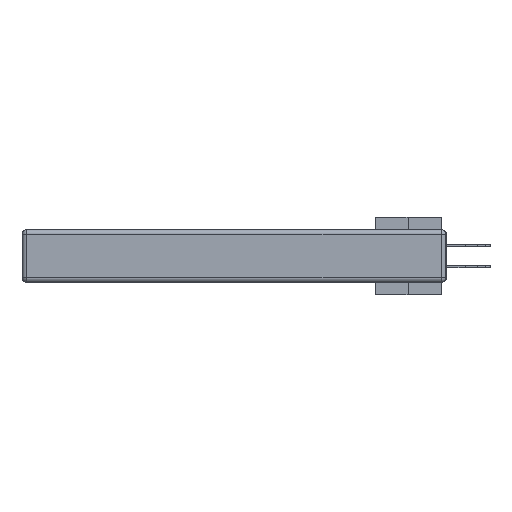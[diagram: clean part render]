
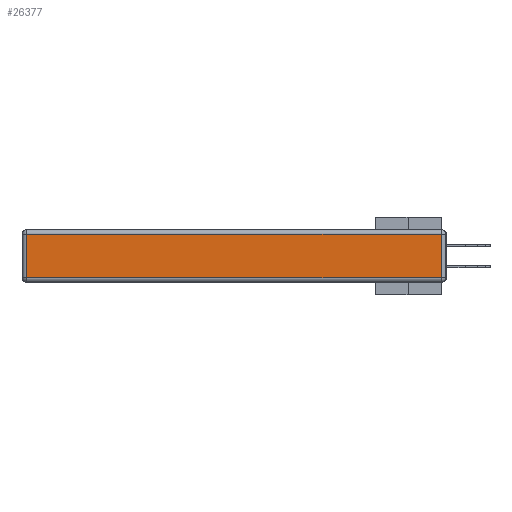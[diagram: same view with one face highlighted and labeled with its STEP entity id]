
A CAD part, left-side view. The second image highlights one B-rep face of the part: STEP entity #26377.
In plain terms, the highlighted planar face has unit normal (-1, 0, 0).
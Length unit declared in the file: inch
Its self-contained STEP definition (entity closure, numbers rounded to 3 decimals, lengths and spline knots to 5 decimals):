
#794 = EDGE_CURVE ( 'NONE', #29100, #9804, #16203, .T. ) ;
#1527 = CARTESIAN_POINT ( 'NONE',  ( 0., 2.75, -0.03 ) ) ;
#2427 = EDGE_LOOP ( 'NONE', ( #33691, #31388, #11139, #40716 ) ) ;
#3184 = CARTESIAN_POINT ( 'NONE',  ( 0., 2.72, -0.03 ) ) ;
#4443 = FACE_OUTER_BOUND ( 'NONE', #2427, .T. ) ;
#7871 = VERTEX_POINT ( 'NONE', #13119 ) ;
#8335 = LINE ( 'NONE', #18877, #35771 ) ;
#8372 = CARTESIAN_POINT ( 'NONE',  ( 0., 2.72, -0.313 ) ) ;
#9804 = VERTEX_POINT ( 'NONE', #3184 ) ;
#10887 = CARTESIAN_POINT ( 'NONE',  ( 0., 0.03, -0.03 ) ) ;
#11139 = ORIENTED_EDGE ( 'NONE', *, *, #794, .T. ) ;
#11229 = EDGE_CURVE ( 'NONE', #7871, #29100, #8335, .T. ) ;
#12417 = VECTOR ( 'NONE', #27567, 39.37008 ) ;
#13119 = CARTESIAN_POINT ( 'NONE',  ( 0., 0.03, -0.313 ) ) ;
#14620 = EDGE_CURVE ( 'NONE', #21224, #7871, #17449, .T. ) ;
#15185 = LINE ( 'NONE', #41942, #37026 ) ;
#16203 = LINE ( 'NONE', #1527, #41329 ) ;
#17449 = LINE ( 'NONE', #35045, #12417 ) ;
#18333 = CARTESIAN_POINT ( 'NONE',  ( 0., 0., -0.343 ) ) ;
#18877 = CARTESIAN_POINT ( 'NONE',  ( 0., 0.03, -0.343 ) ) ;
#21224 = VERTEX_POINT ( 'NONE', #8372 ) ;
#21753 = AXIS2_PLACEMENT_3D ( 'NONE', #18333, #40061, #32373 ) ;
#22513 = DIRECTION ( 'NONE',  ( 0., 0., 1. ) ) ;
#26377 = ADVANCED_FACE ( 'NONE', ( #4443 ), #36484, .T. ) ;
#27567 = DIRECTION ( 'NONE',  ( 0., -1., 0. ) ) ;
#29100 = VERTEX_POINT ( 'NONE', #10887 ) ;
#31388 = ORIENTED_EDGE ( 'NONE', *, *, #11229, .T. ) ;
#32373 = DIRECTION ( 'NONE',  ( 0., 0., 1. ) ) ;
#33691 = ORIENTED_EDGE ( 'NONE', *, *, #14620, .T. ) ;
#33812 = EDGE_CURVE ( 'NONE', #9804, #21224, #15185, .T. ) ;
#35045 = CARTESIAN_POINT ( 'NONE',  ( 0., 0., -0.313 ) ) ;
#35771 = VECTOR ( 'NONE', #22513, 39.37008 ) ;
#36484 = PLANE ( 'NONE',  #21753 ) ;
#37026 = VECTOR ( 'NONE', #41800, 39.37008 ) ;
#40061 = DIRECTION ( 'NONE',  ( -1., 0., 0. ) ) ;
#40716 = ORIENTED_EDGE ( 'NONE', *, *, #33812, .T. ) ;
#40793 = DIRECTION ( 'NONE',  ( 0., 1., 0. ) ) ;
#41329 = VECTOR ( 'NONE', #40793, 39.37008 ) ;
#41800 = DIRECTION ( 'NONE',  ( 0., 0., -1. ) ) ;
#41942 = CARTESIAN_POINT ( 'NONE',  ( 0., 2.72, -0.343 ) ) ;
